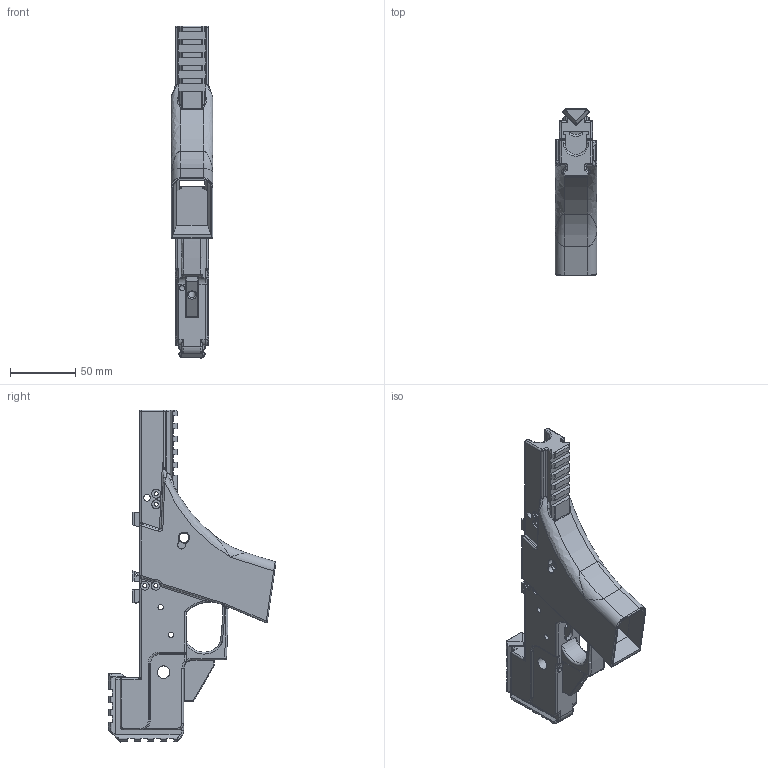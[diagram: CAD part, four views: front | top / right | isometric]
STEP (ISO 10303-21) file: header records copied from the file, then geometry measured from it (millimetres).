
FILE_DESCRIPTION(/* description */ ('RECEIVER'),/* implementation_level */ '2;1');
FILE_NAME(/* name */ '3011DS Standard Barrel.stp',/* time_stamp */ '2022-11-14T10:39:32-06:00',/* author */ ('johne'),/* organization */ (''),/* preprocessor_version */ 'ST-DEVELOPER v19.2',/* originating_system */ 'Autodesk Inventor 2023',/* authorisation */ '');
FILE_SCHEMA (('AUTOMOTIVE_DESIGN { 1 0 10303 214 3 1 1 }'));
Length unit declared in the file: inch
Products named in the file (1): 3011DS Standard Barrel
Bounding box: 32 x 128.88 x 255.05 mm (x, y, z)
Volume: 213100.6 mm3; surface area: 71465.7 mm2
Topology: 1 solids, 1 shells, 740 faces, 1920 edges, 1158 vertices
Faces by surface type: cylinder 275, plane 241, bspline 132, torus 58, sphere 29, cone 5
Full cylindrical faces by diameter (mm): 2.806 x1, 3 x8, 3.518 x1, 4.064 x4, 4.089 x1, 5.105 x2, 5.537 x1, 6.833 x4, 6.845 x2, 7.29 x1, 8.458 x1, 9.652 x2
Entity records: 26669 total; most frequent: CARTESIAN_POINT 8951, ORIENTED_EDGE 3798, DIRECTION 3613, EDGE_CURVE 1899, AXIS2_PLACEMENT_3D 1365, VERTEX_POINT 1158, LINE 883, VECTOR 883
